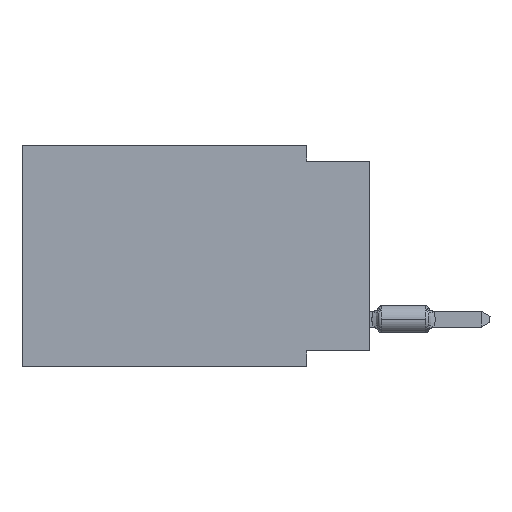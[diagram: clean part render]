
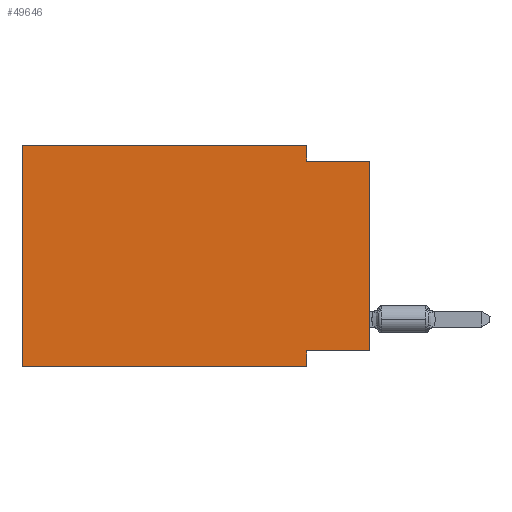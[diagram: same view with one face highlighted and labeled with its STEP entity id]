
A CAD part, left-side view. The second image highlights one B-rep face of the part: STEP entity #49646.
In plain terms, the highlighted planar face has unit normal (-1, 0, 0).
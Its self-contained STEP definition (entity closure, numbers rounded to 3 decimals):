
#1648 = PLANE ( 'NONE',  #105671 ) ;
#3207 = DIRECTION ( 'NONE',  ( 0., -1., 0. ) ) ;
#5961 = EDGE_LOOP ( 'NONE', ( #91656, #81064, #81689, #93028, #47269, #13119, #103224, #88885 ) ) ;
#11286 = DIRECTION ( 'NONE',  ( 0., 1., 0. ) ) ;
#13119 = ORIENTED_EDGE ( 'NONE', *, *, #49690, .T. ) ;
#15842 = LINE ( 'NONE', #51592, #27735 ) ;
#16476 = VECTOR ( 'NONE', #75420, 1000. ) ;
#17743 = EDGE_CURVE ( 'NONE', #52447, #50933, #110787, .T. ) ;
#24786 = DIRECTION ( 'NONE',  ( 0., -1., 0. ) ) ;
#25553 = DIRECTION ( 'NONE',  ( 0., 0., -1. ) ) ;
#25723 = CARTESIAN_POINT ( 'NONE',  ( 0., 2.54, 0. ) ) ;
#27735 = VECTOR ( 'NONE', #24786, 1000. ) ;
#29804 = DIRECTION ( 'NONE',  ( 0., 0., 1. ) ) ;
#31321 = CARTESIAN_POINT ( 'NONE',  ( 0., 13.97, 0. ) ) ;
#34365 = LINE ( 'NONE', #70678, #43895 ) ;
#34603 = VECTOR ( 'NONE', #50066, 1000. ) ;
#34922 = CARTESIAN_POINT ( 'NONE',  ( 0., 0., -0.635 ) ) ;
#35956 = CARTESIAN_POINT ( 'NONE',  ( 0., 13.97, -8.89 ) ) ;
#39268 = CARTESIAN_POINT ( 'NONE',  ( 0., 0., -8.255 ) ) ;
#39532 = CARTESIAN_POINT ( 'NONE',  ( 0., 0., -8.255 ) ) ;
#43895 = VECTOR ( 'NONE', #107011, 1000. ) ;
#47269 = ORIENTED_EDGE ( 'NONE', *, *, #114368, .F. ) ;
#49351 = LINE ( 'NONE', #39268, #102321 ) ;
#49646 = ADVANCED_FACE ( 'NONE', ( #56443 ), #1648, .F. ) ;
#49690 = EDGE_CURVE ( 'NONE', #57537, #52003, #15842, .T. ) ;
#50066 = DIRECTION ( 'NONE',  ( 0., 0., -1. ) ) ;
#50933 = VERTEX_POINT ( 'NONE', #34922 ) ;
#51592 = CARTESIAN_POINT ( 'NONE',  ( 0., 13.97, -8.89 ) ) ;
#52003 = VERTEX_POINT ( 'NONE', #115436 ) ;
#52447 = VERTEX_POINT ( 'NONE', #39532 ) ;
#56443 = FACE_OUTER_BOUND ( 'NONE', #5961, .T. ) ;
#56674 = CARTESIAN_POINT ( 'NONE',  ( 0., 2.54, 0. ) ) ;
#57537 = VERTEX_POINT ( 'NONE', #35956 ) ;
#58408 = LINE ( 'NONE', #56674, #34603 ) ;
#60723 = CARTESIAN_POINT ( 'NONE',  ( 0., 2.54, -0.635 ) ) ;
#65481 = EDGE_CURVE ( 'NONE', #99287, #52003, #107136, .T. ) ;
#70678 = CARTESIAN_POINT ( 'NONE',  ( 0., 0., -0.635 ) ) ;
#74093 = LINE ( 'NONE', #112766, #86089 ) ;
#74301 = DIRECTION ( 'NONE',  ( 1., 0., 0. ) ) ;
#75420 = DIRECTION ( 'NONE',  ( 0., 0., 1. ) ) ;
#76316 = VECTOR ( 'NONE', #29804, 1000. ) ;
#77106 = VECTOR ( 'NONE', #25553, 1000. ) ;
#77156 = LINE ( 'NONE', #31321, #16476 ) ;
#79617 = EDGE_CURVE ( 'NONE', #105236, #50933, #34365, .T. ) ;
#81064 = ORIENTED_EDGE ( 'NONE', *, *, #79617, .F. ) ;
#81610 = CARTESIAN_POINT ( 'NONE',  ( 0., 0., 0. ) ) ;
#81689 = ORIENTED_EDGE ( 'NONE', *, *, #109308, .F. ) ;
#82570 = EDGE_CURVE ( 'NONE', #95811, #87945, #74093, .T. ) ;
#86089 = VECTOR ( 'NONE', #3207, 1000. ) ;
#87945 = VERTEX_POINT ( 'NONE', #25723 ) ;
#88885 = ORIENTED_EDGE ( 'NONE', *, *, #91066, .F. ) ;
#91066 = EDGE_CURVE ( 'NONE', #52447, #99287, #49351, .T. ) ;
#91656 = ORIENTED_EDGE ( 'NONE', *, *, #17743, .T. ) ;
#92752 = CARTESIAN_POINT ( 'NONE',  ( 0., 13.97, 0. ) ) ;
#93028 = ORIENTED_EDGE ( 'NONE', *, *, #82570, .F. ) ;
#95811 = VERTEX_POINT ( 'NONE', #97823 ) ;
#97823 = CARTESIAN_POINT ( 'NONE',  ( 0., 13.97, 0. ) ) ;
#99287 = VERTEX_POINT ( 'NONE', #115247 ) ;
#102321 = VECTOR ( 'NONE', #11286, 1000. ) ;
#103224 = ORIENTED_EDGE ( 'NONE', *, *, #65481, .F. ) ;
#104025 = DIRECTION ( 'NONE',  ( 0., 0., -1. ) ) ;
#105236 = VERTEX_POINT ( 'NONE', #60723 ) ;
#105671 = AXIS2_PLACEMENT_3D ( 'NONE', #92752, #74301, #104025 ) ;
#106552 = CARTESIAN_POINT ( 'NONE',  ( 0., 2.54, -8.89 ) ) ;
#107011 = DIRECTION ( 'NONE',  ( 0., -1., 0. ) ) ;
#107136 = LINE ( 'NONE', #106552, #77106 ) ;
#109308 = EDGE_CURVE ( 'NONE', #87945, #105236, #58408, .T. ) ;
#110787 = LINE ( 'NONE', #81610, #76316 ) ;
#112766 = CARTESIAN_POINT ( 'NONE',  ( 0., 13.97, 0. ) ) ;
#114368 = EDGE_CURVE ( 'NONE', #57537, #95811, #77156, .T. ) ;
#115247 = CARTESIAN_POINT ( 'NONE',  ( 0., 2.54, -8.255 ) ) ;
#115436 = CARTESIAN_POINT ( 'NONE',  ( 0., 2.54, -8.89 ) ) ;
